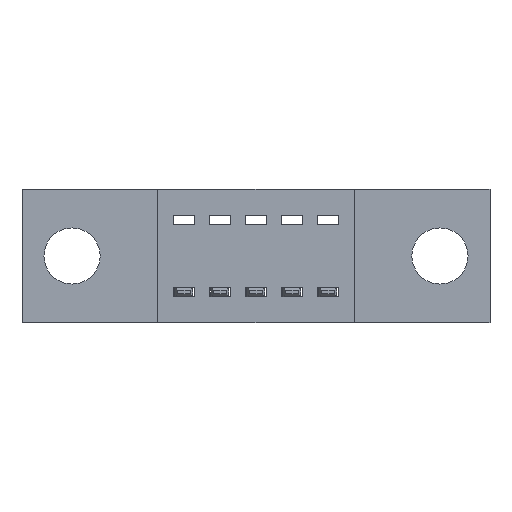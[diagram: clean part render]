
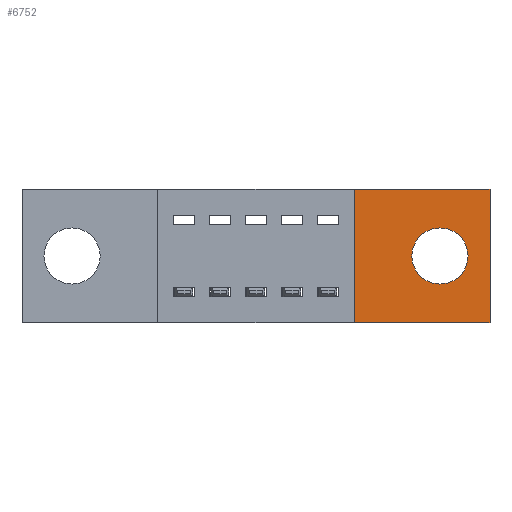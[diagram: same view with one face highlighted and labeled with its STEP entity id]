
A CAD part, front view. The second image highlights one B-rep face of the part: STEP entity #6752.
In plain terms, the highlighted planar face has unit normal (0, -1, 0).
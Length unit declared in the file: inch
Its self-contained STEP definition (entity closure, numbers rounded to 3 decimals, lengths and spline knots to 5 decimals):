
#183 = CIRCLE ( 'NONE', #5515, 0.078 ) ;
#237 = DIRECTION ( 'NONE',  ( 0., 0., -1. ) ) ;
#427 = CARTESIAN_POINT ( 'NONE',  ( 1.3, 0., -0.37 ) ) ;
#521 = VERTEX_POINT ( 'NONE', #6622 ) ;
#554 = EDGE_CURVE ( 'NONE', #1377, #3235, #5470, .T. ) ;
#604 = EDGE_CURVE ( 'NONE', #521, #4035, #5126, .T. ) ;
#652 = AXIS2_PLACEMENT_3D ( 'NONE', #4088, #4080, #4074 ) ;
#885 = ORIENTED_EDGE ( 'NONE', *, *, #4470, .T. ) ;
#909 = EDGE_CURVE ( 'NONE', #3927, #5970, #183, .T. ) ;
#1067 = ORIENTED_EDGE ( 'NONE', *, *, #4371, .F. ) ;
#1377 = VERTEX_POINT ( 'NONE', #6254 ) ;
#1397 = CARTESIAN_POINT ( 'NONE',  ( 1.161, 0., -0.107 ) ) ;
#1606 = CARTESIAN_POINT ( 'NONE',  ( 0.923, 0., -0.37 ) ) ;
#1726 = CARTESIAN_POINT ( 'NONE',  ( 0., 0., 0. ) ) ;
#1868 = EDGE_LOOP ( 'NONE', ( #3833, #885 ) ) ;
#2534 = VECTOR ( 'NONE', #5457, 39.37008 ) ;
#2811 = EDGE_LOOP ( 'NONE', ( #4019, #5525, #7067, #1067 ) ) ;
#2871 = FACE_OUTER_BOUND ( 'NONE', #2811, .T. ) ;
#3235 = VERTEX_POINT ( 'NONE', #427 ) ;
#3249 = DIRECTION ( 'NONE',  ( 0., 0., -1. ) ) ;
#3365 = DIRECTION ( 'NONE',  ( 0., 0., 1. ) ) ;
#3469 = CARTESIAN_POINT ( 'NONE',  ( 1.161, 0., -0.263 ) ) ;
#3833 = ORIENTED_EDGE ( 'NONE', *, *, #909, .T. ) ;
#3927 = VERTEX_POINT ( 'NONE', #1397 ) ;
#4019 = ORIENTED_EDGE ( 'NONE', *, *, #604, .F. ) ;
#4035 = VERTEX_POINT ( 'NONE', #4617 ) ;
#4074 = DIRECTION ( 'NONE',  ( 0., 0., -1. ) ) ;
#4080 = DIRECTION ( 'NONE',  ( 0., -1., 0. ) ) ;
#4088 = CARTESIAN_POINT ( 'NONE',  ( 0., 0., -0.37 ) ) ;
#4095 = PLANE ( 'NONE',  #652 ) ;
#4102 = FACE_BOUND ( 'NONE', #1868, .T. ) ;
#4266 = DIRECTION ( 'NONE',  ( 0., 1., 0. ) ) ;
#4323 = LINE ( 'NONE', #1726, #2534 ) ;
#4371 = EDGE_CURVE ( 'NONE', #4035, #1377, #4323, .T. ) ;
#4411 = EDGE_CURVE ( 'NONE', #3235, #521, #5826, .T. ) ;
#4470 = EDGE_CURVE ( 'NONE', #5970, #3927, #6456, .T. ) ;
#4617 = CARTESIAN_POINT ( 'NONE',  ( 0.923, 0., 0. ) ) ;
#5126 = LINE ( 'NONE', #1606, #6651 ) ;
#5336 = AXIS2_PLACEMENT_3D ( 'NONE', #6092, #4266, #237 ) ;
#5457 = DIRECTION ( 'NONE',  ( 1., 0., 0. ) ) ;
#5470 = LINE ( 'NONE', #7143, #6845 ) ;
#5515 = AXIS2_PLACEMENT_3D ( 'NONE', #6251, #7390, #3249 ) ;
#5525 = ORIENTED_EDGE ( 'NONE', *, *, #4411, .F. ) ;
#5826 = LINE ( 'NONE', #6127, #6824 ) ;
#5970 = VERTEX_POINT ( 'NONE', #3469 ) ;
#6092 = CARTESIAN_POINT ( 'NONE',  ( 1.161, 0., -0.185 ) ) ;
#6127 = CARTESIAN_POINT ( 'NONE',  ( 0., 0., -0.37 ) ) ;
#6194 = DIRECTION ( 'NONE',  ( -1., 0., 0. ) ) ;
#6251 = CARTESIAN_POINT ( 'NONE',  ( 1.161, 0., -0.185 ) ) ;
#6254 = CARTESIAN_POINT ( 'NONE',  ( 1.3, 0., 0. ) ) ;
#6456 = CIRCLE ( 'NONE', #5336, 0.078 ) ;
#6622 = CARTESIAN_POINT ( 'NONE',  ( 0.923, 0., -0.37 ) ) ;
#6651 = VECTOR ( 'NONE', #3365, 39.37008 ) ;
#6752 = ADVANCED_FACE ( 'NONE', ( #4102, #2871 ), #4095, .T. ) ;
#6824 = VECTOR ( 'NONE', #6194, 39.37008 ) ;
#6845 = VECTOR ( 'NONE', #7051, 39.37008 ) ;
#7051 = DIRECTION ( 'NONE',  ( 0., 0., -1. ) ) ;
#7067 = ORIENTED_EDGE ( 'NONE', *, *, #554, .F. ) ;
#7143 = CARTESIAN_POINT ( 'NONE',  ( 1.3, 0., 0. ) ) ;
#7390 = DIRECTION ( 'NONE',  ( 0., 1., 0. ) ) ;
